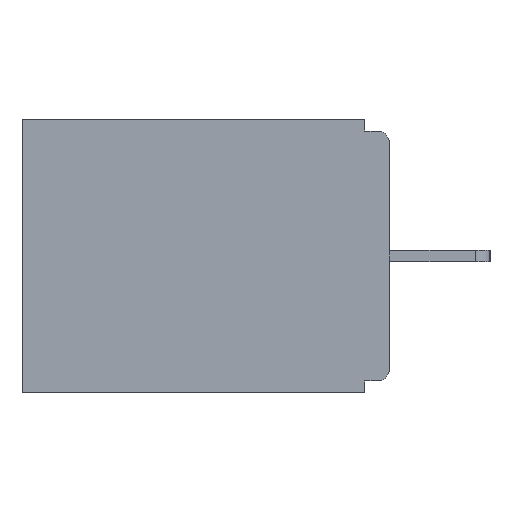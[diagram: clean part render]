
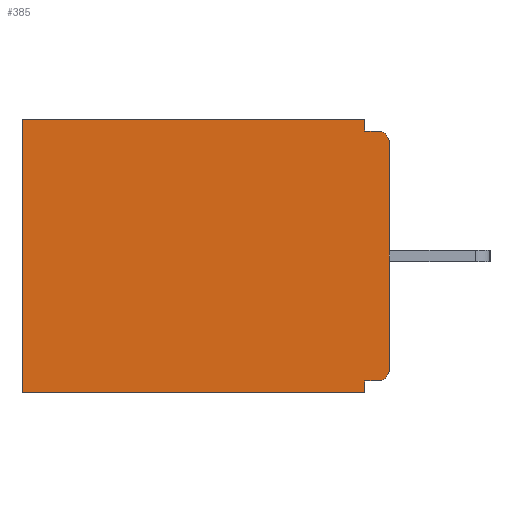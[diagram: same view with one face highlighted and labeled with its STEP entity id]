
A CAD part, left-side view. The second image highlights one B-rep face of the part: STEP entity #385.
In plain terms, the highlighted planar face has unit normal (-1, 0, 0).
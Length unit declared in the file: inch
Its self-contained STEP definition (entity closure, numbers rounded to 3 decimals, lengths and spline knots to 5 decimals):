
#24 = EDGE_LOOP ( 'NONE', ( #4127, #6966, #3311, #6370, #7169, #2508, #348, #7637, #5808, #2870 ) ) ;
#144 = EDGE_CURVE ( 'NONE', #6798, #6265, #6663, .T. ) ;
#254 = VECTOR ( 'NONE', #2024, 39.37008 ) ;
#271 = LINE ( 'NONE', #5870, #254 ) ;
#348 = ORIENTED_EDGE ( 'NONE', *, *, #8114, .F. ) ;
#385 = ADVANCED_FACE ( 'NONE', ( #6149 ), #9421, .F. ) ;
#491 = EDGE_CURVE ( 'NONE', #2337, #6265, #5938, .T. ) ;
#714 = EDGE_CURVE ( 'NONE', #2337, #1465, #5497, .T. ) ;
#992 = LINE ( 'NONE', #5289, #3271 ) ;
#1024 = EDGE_CURVE ( 'NONE', #8925, #7258, #4855, .T. ) ;
#1143 = CARTESIAN_POINT ( 'NONE',  ( 0.298, 0.031, -0.343 ) ) ;
#1387 = VERTEX_POINT ( 'NONE', #7493 ) ;
#1459 = EDGE_CURVE ( 'NONE', #8312, #7668, #3992, .T. ) ;
#1465 = VERTEX_POINT ( 'NONE', #9302 ) ;
#1600 = CARTESIAN_POINT ( 'NONE',  ( 0.298, 0., -0.328 ) ) ;
#1696 = CARTESIAN_POINT ( 'NONE',  ( 0.298, 0.46, 0. ) ) ;
#1835 = DIRECTION ( 'NONE',  ( 0., 0., -1. ) ) ;
#2024 = DIRECTION ( 'NONE',  ( 0., 0., -1. ) ) ;
#2038 = CARTESIAN_POINT ( 'NONE',  ( 0.298, 0.46, 0. ) ) ;
#2210 = DIRECTION ( 'NONE',  ( 1., 0., 0. ) ) ;
#2275 = CARTESIAN_POINT ( 'NONE',  ( 0.298, 0.031, -0.343 ) ) ;
#2337 = VERTEX_POINT ( 'NONE', #7661 ) ;
#2416 = VECTOR ( 'NONE', #8465, 39.37008 ) ;
#2508 = ORIENTED_EDGE ( 'NONE', *, *, #1024, .F. ) ;
#2528 = LINE ( 'NONE', #1600, #2416 ) ;
#2869 = DIRECTION ( 'NONE',  ( 0., 0., -1. ) ) ;
#2870 = ORIENTED_EDGE ( 'NONE', *, *, #491, .F. ) ;
#2918 = VERTEX_POINT ( 'NONE', #8614 ) ;
#2981 = EDGE_CURVE ( 'NONE', #8312, #2918, #271, .T. ) ;
#3028 = CARTESIAN_POINT ( 'NONE',  ( 0.298, 0.015, -0.313 ) ) ;
#3166 = AXIS2_PLACEMENT_3D ( 'NONE', #3028, #3308, #2869 ) ;
#3263 = DIRECTION ( 'NONE',  ( 0., 0., -1. ) ) ;
#3271 = VECTOR ( 'NONE', #4728, 39.37008 ) ;
#3308 = DIRECTION ( 'NONE',  ( -1., 0., 0. ) ) ;
#3311 = ORIENTED_EDGE ( 'NONE', *, *, #2981, .F. ) ;
#3979 = VECTOR ( 'NONE', #9725, 39.37008 ) ;
#3992 = LINE ( 'NONE', #9319, #3979 ) ;
#4024 = AXIS2_PLACEMENT_3D ( 'NONE', #8541, #2210, #3263 ) ;
#4127 = ORIENTED_EDGE ( 'NONE', *, *, #714, .T. ) ;
#4141 = CARTESIAN_POINT ( 'NONE',  ( 0.298, 0.015, -0.328 ) ) ;
#4728 = DIRECTION ( 'NONE',  ( 0., -1., 0. ) ) ;
#4826 = VECTOR ( 'NONE', #8456, 39.37008 ) ;
#4855 = LINE ( 'NONE', #8485, #4826 ) ;
#4955 = EDGE_CURVE ( 'NONE', #6798, #1387, #2528, .T. ) ;
#5167 = CARTESIAN_POINT ( 'NONE',  ( 0.298, 0., -0.313 ) ) ;
#5221 = CARTESIAN_POINT ( 'NONE',  ( 0.298, 0.015, -0.03 ) ) ;
#5251 = DIRECTION ( 'NONE',  ( -1., 0., 0. ) ) ;
#5258 = DIRECTION ( 'NONE',  ( 0., 0., -1. ) ) ;
#5289 = CARTESIAN_POINT ( 'NONE',  ( 0.298, 0., -0.015 ) ) ;
#5497 = CIRCLE ( 'NONE', #5522, 0.015 ) ;
#5522 = AXIS2_PLACEMENT_3D ( 'NONE', #5221, #5251, #5258 ) ;
#5808 = ORIENTED_EDGE ( 'NONE', *, *, #144, .T. ) ;
#5870 = CARTESIAN_POINT ( 'NONE',  ( 0.298, 0.031, -0.343 ) ) ;
#5920 = VECTOR ( 'NONE', #6260, 39.37008 ) ;
#5938 = LINE ( 'NONE', #9349, #5920 ) ;
#6149 = FACE_OUTER_BOUND ( 'NONE', #24, .T. ) ;
#6213 = EDGE_CURVE ( 'NONE', #7668, #7258, #6662, .T. ) ;
#6260 = DIRECTION ( 'NONE',  ( 0., 0., -1. ) ) ;
#6265 = VERTEX_POINT ( 'NONE', #5167 ) ;
#6370 = ORIENTED_EDGE ( 'NONE', *, *, #1459, .T. ) ;
#6629 = VECTOR ( 'NONE', #6905, 39.37008 ) ;
#6662 = LINE ( 'NONE', #1696, #7209 ) ;
#6663 = CIRCLE ( 'NONE', #3166, 0.015 ) ;
#6798 = VERTEX_POINT ( 'NONE', #4141 ) ;
#6905 = DIRECTION ( 'NONE',  ( 0., 0., -1. ) ) ;
#6966 = ORIENTED_EDGE ( 'NONE', *, *, #7154, .F. ) ;
#7154 = EDGE_CURVE ( 'NONE', #2918, #1465, #992, .T. ) ;
#7169 = ORIENTED_EDGE ( 'NONE', *, *, #6213, .T. ) ;
#7209 = VECTOR ( 'NONE', #1835, 39.37008 ) ;
#7258 = VERTEX_POINT ( 'NONE', #8867 ) ;
#7493 = CARTESIAN_POINT ( 'NONE',  ( 0.298, 0.031, -0.328 ) ) ;
#7637 = ORIENTED_EDGE ( 'NONE', *, *, #4955, .F. ) ;
#7661 = CARTESIAN_POINT ( 'NONE',  ( 0.298, 0., -0.03 ) ) ;
#7668 = VERTEX_POINT ( 'NONE', #2038 ) ;
#8114 = EDGE_CURVE ( 'NONE', #1387, #8925, #8309, .T. ) ;
#8309 = LINE ( 'NONE', #1143, #6629 ) ;
#8312 = VERTEX_POINT ( 'NONE', #9222 ) ;
#8456 = DIRECTION ( 'NONE',  ( 0., 1., 0. ) ) ;
#8465 = DIRECTION ( 'NONE',  ( 0., 1., 0. ) ) ;
#8485 = CARTESIAN_POINT ( 'NONE',  ( 0.298, 0., -0.343 ) ) ;
#8541 = CARTESIAN_POINT ( 'NONE',  ( 0.298, 0., 0. ) ) ;
#8614 = CARTESIAN_POINT ( 'NONE',  ( 0.298, 0.031, -0.015 ) ) ;
#8867 = CARTESIAN_POINT ( 'NONE',  ( 0.298, 0.46, -0.343 ) ) ;
#8925 = VERTEX_POINT ( 'NONE', #2275 ) ;
#9222 = CARTESIAN_POINT ( 'NONE',  ( 0.298, 0.031, 0. ) ) ;
#9302 = CARTESIAN_POINT ( 'NONE',  ( 0.298, 0.015, -0.015 ) ) ;
#9319 = CARTESIAN_POINT ( 'NONE',  ( 0.298, 0., 0. ) ) ;
#9349 = CARTESIAN_POINT ( 'NONE',  ( 0.298, 0., 0. ) ) ;
#9421 = PLANE ( 'NONE',  #4024 ) ;
#9725 = DIRECTION ( 'NONE',  ( 0., 1., 0. ) ) ;
